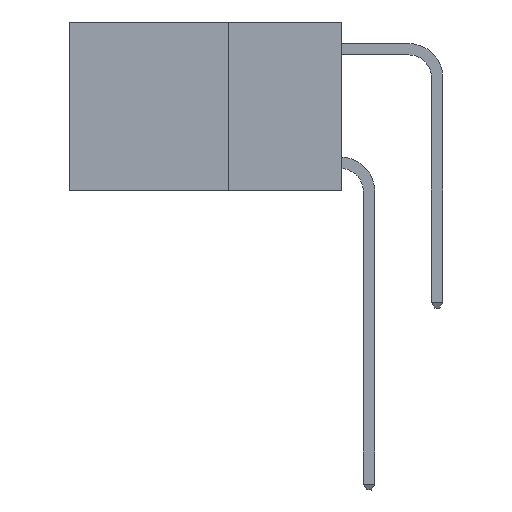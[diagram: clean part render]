
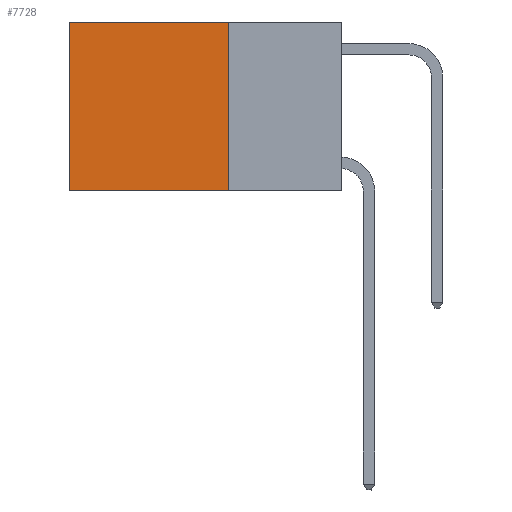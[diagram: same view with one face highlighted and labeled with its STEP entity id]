
A CAD part, left-side view. The second image highlights one B-rep face of the part: STEP entity #7728.
In plain terms, the highlighted planar face has unit normal (-1, 0, 0).
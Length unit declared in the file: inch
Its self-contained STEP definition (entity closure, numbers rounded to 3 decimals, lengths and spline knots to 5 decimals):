
#1029 = CARTESIAN_POINT ( 'NONE',  ( 0.2625, 0.6, 0. ) ) ;
#1788 = CARTESIAN_POINT ( 'NONE',  ( 0.2625, 0.25, 0. ) ) ;
#2978 = CARTESIAN_POINT ( 'NONE',  ( 0.2625, 0.25, -0.37 ) ) ;
#3515 = VERTEX_POINT ( 'NONE', #6381 ) ;
#3542 = DIRECTION ( 'NONE',  ( 1., 0., 0. ) ) ;
#3617 = ORIENTED_EDGE ( 'NONE', *, *, #21441, .T. ) ;
#4164 = LINE ( 'NONE', #13389, #8272 ) ;
#4555 = VERTEX_POINT ( 'NONE', #1029 ) ;
#5864 = LINE ( 'NONE', #16873, #9971 ) ;
#6381 = CARTESIAN_POINT ( 'NONE',  ( 0.2625, 0.25, 0. ) ) ;
#6541 = CARTESIAN_POINT ( 'NONE',  ( 0.2625, 0.25, 0. ) ) ;
#6578 = EDGE_CURVE ( 'NONE', #15815, #17305, #5864, .T. ) ;
#7728 = ADVANCED_FACE ( 'NONE', ( #9640 ), #12270, .F. ) ;
#8272 = VECTOR ( 'NONE', #22084, 39.37008 ) ;
#8505 = LINE ( 'NONE', #6541, #13962 ) ;
#9640 = FACE_OUTER_BOUND ( 'NONE', #13174, .T. ) ;
#9712 = ORIENTED_EDGE ( 'NONE', *, *, #6578, .F. ) ;
#9971 = VECTOR ( 'NONE', #18635, 39.37008 ) ;
#12270 = PLANE ( 'NONE',  #19165 ) ;
#13174 = EDGE_LOOP ( 'NONE', ( #3617, #9712, #14770, #20411 ) ) ;
#13389 = CARTESIAN_POINT ( 'NONE',  ( 0.2625, 0.25, 0. ) ) ;
#13902 = CARTESIAN_POINT ( 'NONE',  ( 0.2625, 0.6, 0. ) ) ;
#13962 = VECTOR ( 'NONE', #16987, 39.37008 ) ;
#14770 = ORIENTED_EDGE ( 'NONE', *, *, #18203, .F. ) ;
#15654 = DIRECTION ( 'NONE',  ( 0., 0., -1. ) ) ;
#15805 = DIRECTION ( 'NONE',  ( 0., 0., -1. ) ) ;
#15815 = VERTEX_POINT ( 'NONE', #2978 ) ;
#16873 = CARTESIAN_POINT ( 'NONE',  ( 0.2625, 0.25, -0.37 ) ) ;
#16874 = LINE ( 'NONE', #13902, #22065 ) ;
#16987 = DIRECTION ( 'NONE',  ( 0., 1., 0. ) ) ;
#17305 = VERTEX_POINT ( 'NONE', #21647 ) ;
#18203 = EDGE_CURVE ( 'NONE', #3515, #15815, #4164, .T. ) ;
#18635 = DIRECTION ( 'NONE',  ( 0., 1., 0. ) ) ;
#19165 = AXIS2_PLACEMENT_3D ( 'NONE', #1788, #3542, #15805 ) ;
#20016 = EDGE_CURVE ( 'NONE', #3515, #4555, #8505, .T. ) ;
#20411 = ORIENTED_EDGE ( 'NONE', *, *, #20016, .T. ) ;
#21441 = EDGE_CURVE ( 'NONE', #4555, #17305, #16874, .T. ) ;
#21647 = CARTESIAN_POINT ( 'NONE',  ( 0.2625, 0.6, -0.37 ) ) ;
#22065 = VECTOR ( 'NONE', #15654, 39.37008 ) ;
#22084 = DIRECTION ( 'NONE',  ( 0., 0., -1. ) ) ;
